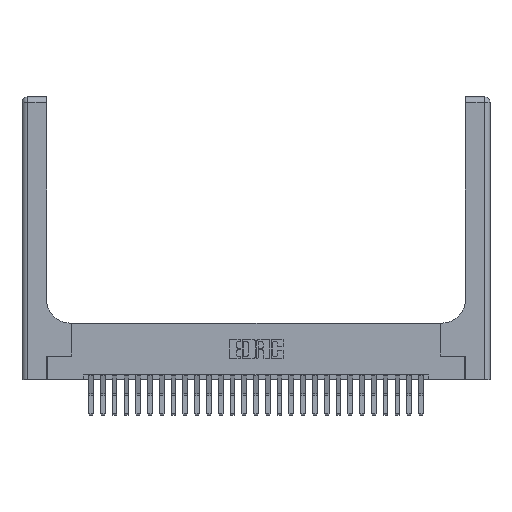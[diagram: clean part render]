
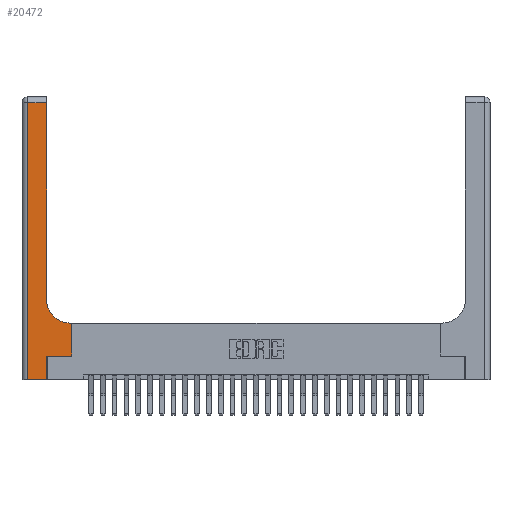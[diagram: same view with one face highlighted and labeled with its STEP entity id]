
A CAD part, top view. The second image highlights one B-rep face of the part: STEP entity #20472.
In plain terms, the highlighted planar face has unit normal (0, 0, 1).
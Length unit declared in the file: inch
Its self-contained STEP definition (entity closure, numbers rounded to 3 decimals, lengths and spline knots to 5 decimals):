
#196 = VERTEX_POINT ( 'NONE', #22458 ) ;
#705 = DIRECTION ( 'NONE',  ( 0., 0., -1. ) ) ;
#1701 = VECTOR ( 'NONE', #3167, 39.37008 ) ;
#2043 = EDGE_CURVE ( 'NONE', #20207, #22693, #6753, .T. ) ;
#2064 = CARTESIAN_POINT ( 'NONE',  ( 0.26, 2.94, 0.37 ) ) ;
#2255 = DIRECTION ( 'NONE',  ( 1., 0., 0. ) ) ;
#2383 = CARTESIAN_POINT ( 'NONE',  ( 0.06, 2.94, 0.37 ) ) ;
#2584 = AXIS2_PLACEMENT_3D ( 'NONE', #17063, #17329, #7147 ) ;
#3167 = DIRECTION ( 'NONE',  ( 0., 1., 0. ) ) ;
#3366 = ORIENTED_EDGE ( 'NONE', *, *, #24601, .T. ) ;
#3757 = ORIENTED_EDGE ( 'NONE', *, *, #13354, .T. ) ;
#3923 = ORIENTED_EDGE ( 'NONE', *, *, #2043, .T. ) ;
#3937 = ORIENTED_EDGE ( 'NONE', *, *, #19038, .T. ) ;
#3963 = CIRCLE ( 'NONE', #18906, 0.25 ) ;
#4253 = EDGE_CURVE ( 'NONE', #17459, #11429, #21557, .T. ) ;
#4753 = PLANE ( 'NONE',  #2584 ) ;
#5135 = LINE ( 'NONE', #17185, #12027 ) ;
#5231 = DIRECTION ( 'NONE',  ( -1., 0., 0. ) ) ;
#5369 = VECTOR ( 'NONE', #21167, 39.37008 ) ;
#5493 = ORIENTED_EDGE ( 'NONE', *, *, #22887, .T. ) ;
#5532 = DIRECTION ( 'NONE',  ( 1., 0., 0. ) ) ;
#6749 = CARTESIAN_POINT ( 'NONE',  ( 0.265, 0.25, 0.37 ) ) ;
#6753 = LINE ( 'NONE', #21212, #1701 ) ;
#7147 = DIRECTION ( 'NONE',  ( -1., 0., 0. ) ) ;
#8116 = LINE ( 'NONE', #10651, #21315 ) ;
#8457 = EDGE_CURVE ( 'NONE', #22693, #23432, #12990, .T. ) ;
#8548 = ORIENTED_EDGE ( 'NONE', *, *, #4253, .T. ) ;
#8677 = CARTESIAN_POINT ( 'NONE',  ( 0.51, 0.6, 0.37 ) ) ;
#8973 = VERTEX_POINT ( 'NONE', #8677 ) ;
#9619 = VECTOR ( 'NONE', #5532, 39.37008 ) ;
#9768 = CARTESIAN_POINT ( 'NONE',  ( 0.06, 0., 0.37 ) ) ;
#10034 = EDGE_CURVE ( 'NONE', #21739, #17459, #21844, .T. ) ;
#10651 = CARTESIAN_POINT ( 'NONE',  ( 0., 0., 0.37 ) ) ;
#11429 = VERTEX_POINT ( 'NONE', #20799 ) ;
#11506 = LINE ( 'NONE', #15404, #22145 ) ;
#11601 = CARTESIAN_POINT ( 'NONE',  ( 0.06, 3., 0.37 ) ) ;
#11722 = CARTESIAN_POINT ( 'NONE',  ( 0.26, 0.85, 0.37 ) ) ;
#12027 = VECTOR ( 'NONE', #23055, 39.37008 ) ;
#12060 = CARTESIAN_POINT ( 'NONE',  ( 0.265, 0.25, 0.37 ) ) ;
#12839 = ORIENTED_EDGE ( 'NONE', *, *, #18426, .T. ) ;
#12990 = LINE ( 'NONE', #17291, #5369 ) ;
#13354 = EDGE_CURVE ( 'NONE', #23432, #15827, #21782, .T. ) ;
#13372 = EDGE_LOOP ( 'NONE', ( #3923, #14089, #3757, #3937, #3366, #25492, #8548, #12839, #5493 ) ) ;
#14089 = ORIENTED_EDGE ( 'NONE', *, *, #8457, .T. ) ;
#14362 = VECTOR ( 'NONE', #23916, 39.37008 ) ;
#15134 = CARTESIAN_POINT ( 'NONE',  ( 0.51, 0.85, 0.37 ) ) ;
#15404 = CARTESIAN_POINT ( 'NONE',  ( 0.26, 0.6, 0.37 ) ) ;
#15827 = VERTEX_POINT ( 'NONE', #9768 ) ;
#17063 = CARTESIAN_POINT ( 'NONE',  ( 0., 3., 0.37 ) ) ;
#17185 = CARTESIAN_POINT ( 'NONE',  ( 0.265, 0., 0.37 ) ) ;
#17291 = CARTESIAN_POINT ( 'NONE',  ( 0., 2.94, 0.37 ) ) ;
#17329 = DIRECTION ( 'NONE',  ( 0., 0., -1. ) ) ;
#17459 = VERTEX_POINT ( 'NONE', #25965 ) ;
#18426 = EDGE_CURVE ( 'NONE', #11429, #8973, #11506, .T. ) ;
#18906 = AXIS2_PLACEMENT_3D ( 'NONE', #15134, #705, #19289 ) ;
#19038 = EDGE_CURVE ( 'NONE', #15827, #196, #8116, .T. ) ;
#19289 = DIRECTION ( 'NONE',  ( 1., 0., 0. ) ) ;
#20207 = VERTEX_POINT ( 'NONE', #11722 ) ;
#20472 = ADVANCED_FACE ( 'NONE', ( #21466 ), #4753, .F. ) ;
#20799 = CARTESIAN_POINT ( 'NONE',  ( 0.528, 0.6, 0.37 ) ) ;
#21167 = DIRECTION ( 'NONE',  ( -1., 0., 0. ) ) ;
#21212 = CARTESIAN_POINT ( 'NONE',  ( 0.26, 3., 0.37 ) ) ;
#21315 = VECTOR ( 'NONE', #2255, 39.37008 ) ;
#21466 = FACE_OUTER_BOUND ( 'NONE', #13372, .T. ) ;
#21557 = LINE ( 'NONE', #23549, #24728 ) ;
#21739 = VERTEX_POINT ( 'NONE', #6749 ) ;
#21782 = LINE ( 'NONE', #11601, #14362 ) ;
#21844 = LINE ( 'NONE', #12060, #9619 ) ;
#22145 = VECTOR ( 'NONE', #5231, 39.37008 ) ;
#22458 = CARTESIAN_POINT ( 'NONE',  ( 0.265, 0., 0.37 ) ) ;
#22693 = VERTEX_POINT ( 'NONE', #2064 ) ;
#22887 = EDGE_CURVE ( 'NONE', #8973, #20207, #3963, .T. ) ;
#23055 = DIRECTION ( 'NONE',  ( 0., 1., 0. ) ) ;
#23432 = VERTEX_POINT ( 'NONE', #2383 ) ;
#23549 = CARTESIAN_POINT ( 'NONE',  ( 0.528, 0.25, 0.37 ) ) ;
#23916 = DIRECTION ( 'NONE',  ( 0., -1., 0. ) ) ;
#24601 = EDGE_CURVE ( 'NONE', #196, #21739, #5135, .T. ) ;
#24728 = VECTOR ( 'NONE', #25975, 39.37008 ) ;
#25492 = ORIENTED_EDGE ( 'NONE', *, *, #10034, .T. ) ;
#25965 = CARTESIAN_POINT ( 'NONE',  ( 0.528, 0.25, 0.37 ) ) ;
#25975 = DIRECTION ( 'NONE',  ( 0., 1., 0. ) ) ;
